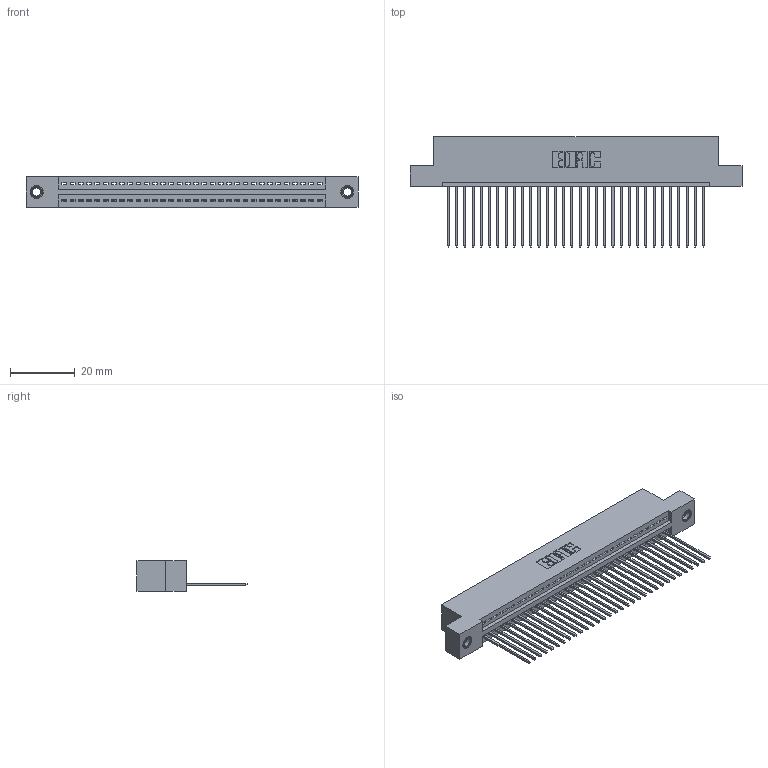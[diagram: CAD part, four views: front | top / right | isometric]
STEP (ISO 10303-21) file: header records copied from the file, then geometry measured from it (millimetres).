
FILE_DESCRIPTION (( 'STEP AP203' ), '1' );
FILE_NAME ('395-032-541-107.STEP', '2019-10-19T14:29:35', ( '' ), ( '' ), 'SwSTEP 2.0', 'SolidWorks 2016', '' );
FILE_SCHEMA (( 'CONFIG_CONTROL_DESIGN' ));
Length unit declared in the file: inch
Products named in the file (4): 395-032-541-107; 345 Part_Flush Mounting Lugs - 0.156 Dia-TI; 345-250-001_345-250-005-103; 345-292-001_345-293-141
Assembly tree (35 placements, depth 2):
  395-032-541-107
    345 Part_Flush Mounting Lugs - 0.156 Dia-TI
    345-292-001_345-293-141  x32
    345-250-001_345-250-005-103  x2
Bounding box: 102.49 x 33.96 x 9.4 mm (x, y, z)
Volume: 9744.7 mm3; surface area: 13467.8 mm2
Topology: 35 solids, 35 shells, 2042 faces, 6109 edges, 4022 vertices
Faces by surface type: plane 1392, cylinder 634, cone 12, torus 4
Entity records: 26634 total; most frequent: CARTESIAN_POINT 4595, ORIENTED_EDGE 4554, DIRECTION 4055, EDGE_CURVE 2277, VECTOR 1997, LINE 1997, VERTEX_POINT 1512, AXIS2_PLACEMENT_3D 1029
